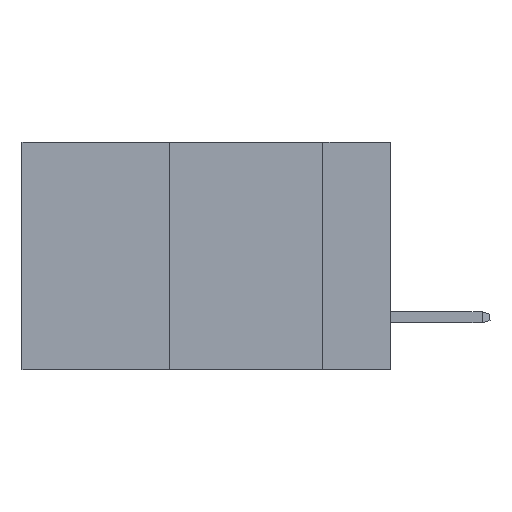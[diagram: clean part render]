
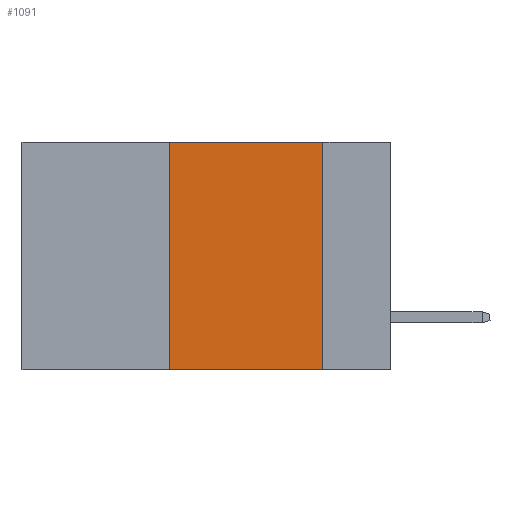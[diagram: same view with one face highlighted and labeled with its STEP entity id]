
A CAD part, left-side view. The second image highlights one B-rep face of the part: STEP entity #1091.
In plain terms, the highlighted planar face has unit normal (-1, 0, 0).
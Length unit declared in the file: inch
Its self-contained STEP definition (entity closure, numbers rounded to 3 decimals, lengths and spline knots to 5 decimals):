
#303 = ORIENTED_EDGE ( 'NONE', *, *, #12078, .T. ) ;
#447 = LINE ( 'NONE', #19332, #12917 ) ;
#1091 = ADVANCED_FACE ( 'NONE', ( #4369 ), #17712, .F. ) ;
#1700 = VECTOR ( 'NONE', #22244, 39.37008 ) ;
#1739 = VERTEX_POINT ( 'NONE', #5853 ) ;
#2120 = EDGE_CURVE ( 'NONE', #6552, #1739, #12718, .T. ) ;
#2455 = CARTESIAN_POINT ( 'NONE',  ( 0., 0.11, 0. ) ) ;
#2842 = VECTOR ( 'NONE', #11626, 39.37008 ) ;
#2966 = EDGE_CURVE ( 'NONE', #19701, #6552, #13237, .T. ) ;
#3178 = AXIS2_PLACEMENT_3D ( 'NONE', #9749, #8424, #13863 ) ;
#3907 = ORIENTED_EDGE ( 'NONE', *, *, #2966, .F. ) ;
#4319 = LINE ( 'NONE', #2455, #13546 ) ;
#4356 = DIRECTION ( 'NONE',  ( 0., 0., -1. ) ) ;
#4369 = FACE_OUTER_BOUND ( 'NONE', #22301, .T. ) ;
#5853 = CARTESIAN_POINT ( 'NONE',  ( 0., 0.11, 0. ) ) ;
#6552 = VERTEX_POINT ( 'NONE', #7181 ) ;
#7181 = CARTESIAN_POINT ( 'NONE',  ( 0., 0.36, 0. ) ) ;
#8424 = DIRECTION ( 'NONE',  ( 1., 0., 0. ) ) ;
#9749 = CARTESIAN_POINT ( 'NONE',  ( 0., 0.6, 0. ) ) ;
#10876 = EDGE_CURVE ( 'NONE', #1739, #19450, #4319, .T. ) ;
#11066 = CARTESIAN_POINT ( 'NONE',  ( 0., 0.11, -0.37 ) ) ;
#11626 = DIRECTION ( 'NONE',  ( 0., 0., 1. ) ) ;
#12025 = DIRECTION ( 'NONE',  ( 0., -1., 0. ) ) ;
#12078 = EDGE_CURVE ( 'NONE', #19701, #19450, #447, .T. ) ;
#12208 = ORIENTED_EDGE ( 'NONE', *, *, #2120, .F. ) ;
#12718 = LINE ( 'NONE', #13691, #1700 ) ;
#12917 = VECTOR ( 'NONE', #12025, 39.37008 ) ;
#13237 = LINE ( 'NONE', #20763, #2842 ) ;
#13546 = VECTOR ( 'NONE', #4356, 39.37008 ) ;
#13626 = CARTESIAN_POINT ( 'NONE',  ( 0., 0.36, -0.37 ) ) ;
#13691 = CARTESIAN_POINT ( 'NONE',  ( 0., 0.6, 0. ) ) ;
#13860 = ORIENTED_EDGE ( 'NONE', *, *, #10876, .F. ) ;
#13863 = DIRECTION ( 'NONE',  ( 0., 0., -1. ) ) ;
#17712 = PLANE ( 'NONE',  #3178 ) ;
#19332 = CARTESIAN_POINT ( 'NONE',  ( 0., 0.6, -0.37 ) ) ;
#19450 = VERTEX_POINT ( 'NONE', #11066 ) ;
#19701 = VERTEX_POINT ( 'NONE', #13626 ) ;
#20763 = CARTESIAN_POINT ( 'NONE',  ( 0., 0.36, 0. ) ) ;
#22244 = DIRECTION ( 'NONE',  ( 0., -1., 0. ) ) ;
#22301 = EDGE_LOOP ( 'NONE', ( #13860, #12208, #3907, #303 ) ) ;
